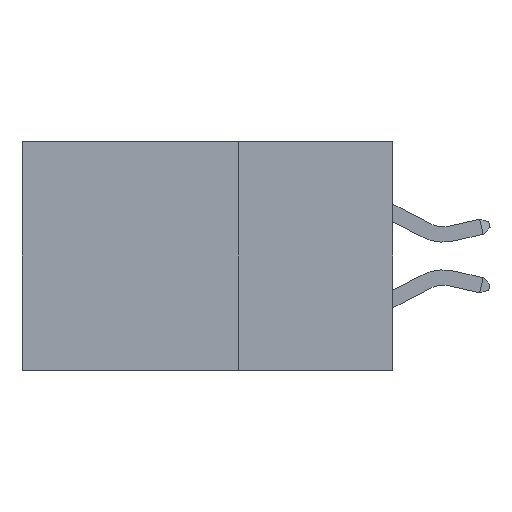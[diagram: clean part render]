
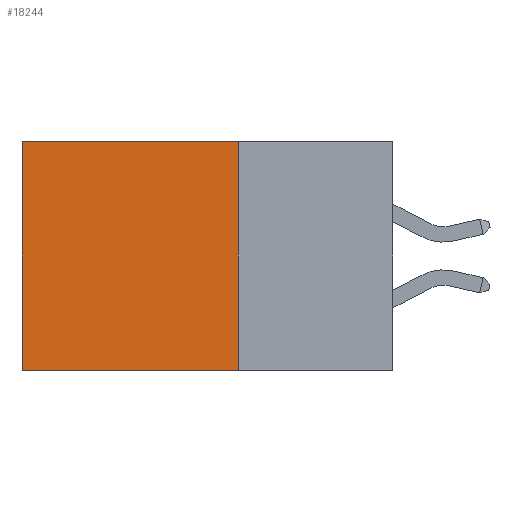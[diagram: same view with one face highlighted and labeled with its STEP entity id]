
A CAD part, left-side view. The second image highlights one B-rep face of the part: STEP entity #18244.
In plain terms, the highlighted planar face has unit normal (-1, 0, 0).
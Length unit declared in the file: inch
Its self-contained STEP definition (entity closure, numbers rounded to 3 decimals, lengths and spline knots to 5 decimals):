
#2176 = LINE ( 'NONE', #15370, #23451 ) ;
#2928 = ORIENTED_EDGE ( 'NONE', *, *, #18145, .F. ) ;
#4644 = LINE ( 'NONE', #17409, #29728 ) ;
#5285 = FACE_OUTER_BOUND ( 'NONE', #15266, .T. ) ;
#6836 = ORIENTED_EDGE ( 'NONE', *, *, #35942, .T. ) ;
#7527 = ORIENTED_EDGE ( 'NONE', *, *, #17378, .F. ) ;
#7823 = CARTESIAN_POINT ( 'NONE',  ( 0.2875, 0.6, -0.37 ) ) ;
#8542 = VECTOR ( 'NONE', #30451, 39.37008 ) ;
#11546 = CARTESIAN_POINT ( 'NONE',  ( 0.2875, 0.6, 0. ) ) ;
#14586 = CARTESIAN_POINT ( 'NONE',  ( 0.2875, 0.6, 0. ) ) ;
#15016 = DIRECTION ( 'NONE',  ( 0., 0., -1. ) ) ;
#15266 = EDGE_LOOP ( 'NONE', ( #6836, #2928, #7527, #38496 ) ) ;
#15370 = CARTESIAN_POINT ( 'NONE',  ( 0.2875, 0.25, 0. ) ) ;
#17026 = CARTESIAN_POINT ( 'NONE',  ( 0.2875, 0.25, -0.37 ) ) ;
#17159 = VERTEX_POINT ( 'NONE', #7823 ) ;
#17378 = EDGE_CURVE ( 'NONE', #28940, #41065, #2176, .T. ) ;
#17409 = CARTESIAN_POINT ( 'NONE',  ( 0.2875, 0.25, -0.37 ) ) ;
#18145 = EDGE_CURVE ( 'NONE', #41065, #17159, #4644, .T. ) ;
#18148 = VERTEX_POINT ( 'NONE', #14586 ) ;
#18244 = ADVANCED_FACE ( 'NONE', ( #5285 ), #25612, .F. ) ;
#18263 = DIRECTION ( 'NONE',  ( 1., 0., 0. ) ) ;
#23306 = EDGE_CURVE ( 'NONE', #28940, #18148, #37349, .T. ) ;
#23451 = VECTOR ( 'NONE', #41768, 39.37008 ) ;
#24245 = CARTESIAN_POINT ( 'NONE',  ( 0.2875, 0.25, 0. ) ) ;
#25612 = PLANE ( 'NONE',  #26949 ) ;
#26949 = AXIS2_PLACEMENT_3D ( 'NONE', #41818, #18263, #15016 ) ;
#27629 = CARTESIAN_POINT ( 'NONE',  ( 0.2875, 0.25, 0. ) ) ;
#27822 = DIRECTION ( 'NONE',  ( 0., 1., 0. ) ) ;
#28232 = LINE ( 'NONE', #11546, #35639 ) ;
#28940 = VERTEX_POINT ( 'NONE', #24245 ) ;
#29728 = VECTOR ( 'NONE', #27822, 39.37008 ) ;
#30451 = DIRECTION ( 'NONE',  ( 0., 1., 0. ) ) ;
#31485 = DIRECTION ( 'NONE',  ( 0., 0., -1. ) ) ;
#35639 = VECTOR ( 'NONE', #31485, 39.37008 ) ;
#35942 = EDGE_CURVE ( 'NONE', #18148, #17159, #28232, .T. ) ;
#37349 = LINE ( 'NONE', #27629, #8542 ) ;
#38496 = ORIENTED_EDGE ( 'NONE', *, *, #23306, .T. ) ;
#41065 = VERTEX_POINT ( 'NONE', #17026 ) ;
#41768 = DIRECTION ( 'NONE',  ( 0., 0., -1. ) ) ;
#41818 = CARTESIAN_POINT ( 'NONE',  ( 0.2875, 0.25, 0. ) ) ;
